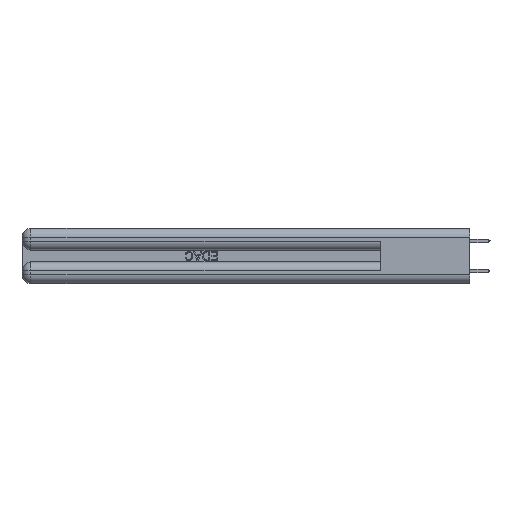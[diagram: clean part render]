
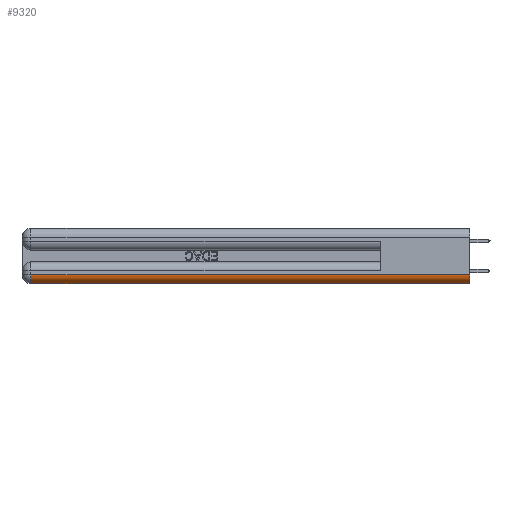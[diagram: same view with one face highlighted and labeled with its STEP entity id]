
A CAD part, left-side view. The second image highlights one B-rep face of the part: STEP entity #9320.
In plain terms, the highlighted cylindrical face has radius 1.524 mm (diameter 3.048 mm), a partial arc.
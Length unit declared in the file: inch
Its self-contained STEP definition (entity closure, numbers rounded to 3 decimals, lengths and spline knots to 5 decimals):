
#325 = DIRECTION ( 'NONE',  ( 0., 1., 0. ) ) ;
#2377 = DIRECTION ( 'NONE',  ( 0., 1., 0. ) ) ;
#3001 = DIRECTION ( 'NONE',  ( 0., 1., 0. ) ) ;
#7038 = EDGE_CURVE ( 'NONE', #7751, #27629, #37576, .T. ) ;
#7751 = VERTEX_POINT ( 'NONE', #23335 ) ;
#8097 = AXIS2_PLACEMENT_3D ( 'NONE', #26185, #3001, #30087 ) ;
#9320 = ADVANCED_FACE ( 'NONE', ( #39755 ), #19233, .T. ) ;
#9922 = ORIENTED_EDGE ( 'NONE', *, *, #7038, .F. ) ;
#11011 = CARTESIAN_POINT ( 'NONE',  ( 0., 0., 0.06 ) ) ;
#12771 = CIRCLE ( 'NONE', #25338, 0.06 ) ;
#14565 = VECTOR ( 'NONE', #21521, 39.37008 ) ;
#19233 = CYLINDRICAL_SURFACE ( 'NONE', #24915, 0.06 ) ;
#19288 = CARTESIAN_POINT ( 'NONE',  ( 0., 2.94, 0.06 ) ) ;
#19588 = CARTESIAN_POINT ( 'NONE',  ( 0.06, 0., 0.06 ) ) ;
#21521 = DIRECTION ( 'NONE',  ( 0., -1., 0. ) ) ;
#23335 = CARTESIAN_POINT ( 'NONE',  ( 0.06, 0., 0. ) ) ;
#23466 = CARTESIAN_POINT ( 'NONE',  ( 0.06, 3., 0. ) ) ;
#23495 = DIRECTION ( 'NONE',  ( 0., 0., 1. ) ) ;
#24867 = LINE ( 'NONE', #40710, #14565 ) ;
#24915 = AXIS2_PLACEMENT_3D ( 'NONE', #25537, #2377, #40990 ) ;
#25338 = AXIS2_PLACEMENT_3D ( 'NONE', #19588, #46501, #23495 ) ;
#25537 = CARTESIAN_POINT ( 'NONE',  ( 0.06, 0., 0.06 ) ) ;
#26185 = CARTESIAN_POINT ( 'NONE',  ( 0.06, 2.94, 0.06 ) ) ;
#26362 = ORIENTED_EDGE ( 'NONE', *, *, #32110, .F. ) ;
#27629 = VERTEX_POINT ( 'NONE', #37625 ) ;
#29181 = VERTEX_POINT ( 'NONE', #11011 ) ;
#29345 = ORIENTED_EDGE ( 'NONE', *, *, #36291, .F. ) ;
#30087 = DIRECTION ( 'NONE',  ( 0., 0., 1. ) ) ;
#31691 = EDGE_LOOP ( 'NONE', ( #26362, #29345, #48819, #9922 ) ) ;
#32110 = EDGE_CURVE ( 'NONE', #29181, #7751, #12771, .T. ) ;
#35444 = CIRCLE ( 'NONE', #8097, 0.06 ) ;
#36291 = EDGE_CURVE ( 'NONE', #46989, #29181, #24867, .T. ) ;
#37576 = LINE ( 'NONE', #23466, #46578 ) ;
#37625 = CARTESIAN_POINT ( 'NONE',  ( 0.06, 2.94, 0. ) ) ;
#38412 = EDGE_CURVE ( 'NONE', #27629, #46989, #35444, .T. ) ;
#39755 = FACE_OUTER_BOUND ( 'NONE', #31691, .T. ) ;
#40710 = CARTESIAN_POINT ( 'NONE',  ( 0., 0., 0.06 ) ) ;
#40990 = DIRECTION ( 'NONE',  ( 0., 0., 1. ) ) ;
#46501 = DIRECTION ( 'NONE',  ( 0., -1., 0. ) ) ;
#46578 = VECTOR ( 'NONE', #325, 39.37008 ) ;
#46989 = VERTEX_POINT ( 'NONE', #19288 ) ;
#48819 = ORIENTED_EDGE ( 'NONE', *, *, #38412, .F. ) ;
